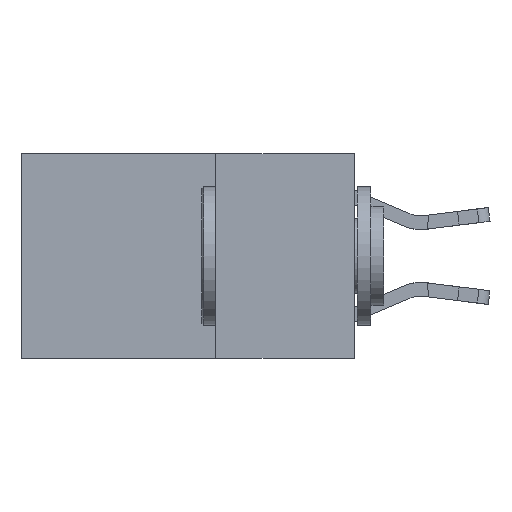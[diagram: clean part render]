
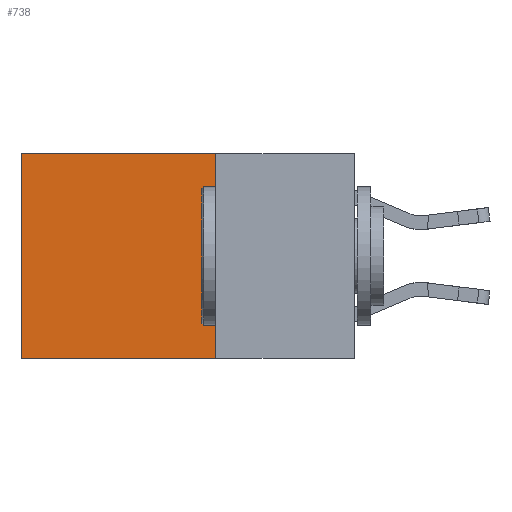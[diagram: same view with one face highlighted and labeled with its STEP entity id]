
A CAD part, left-side view. The second image highlights one B-rep face of the part: STEP entity #738.
In plain terms, the highlighted planar face has unit normal (-1, 0, 0).
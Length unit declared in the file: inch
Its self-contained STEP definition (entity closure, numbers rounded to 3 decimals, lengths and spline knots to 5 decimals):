
#284 = VERTEX_POINT ( 'NONE', #6397 ) ;
#473 = EDGE_LOOP ( 'NONE', ( #6124, #10874, #9040, #774 ) ) ;
#738 = ADVANCED_FACE ( 'NONE', ( #1685 ), #13209, .F. ) ;
#774 = ORIENTED_EDGE ( 'NONE', *, *, #2494, .T. ) ;
#1008 = CARTESIAN_POINT ( 'NONE',  ( 0.2625, 0.6, -0.37 ) ) ;
#1358 = DIRECTION ( 'NONE',  ( 0., 0., -1. ) ) ;
#1457 = CARTESIAN_POINT ( 'NONE',  ( 0.2625, 0.6, 0. ) ) ;
#1685 = FACE_OUTER_BOUND ( 'NONE', #473, .T. ) ;
#2107 = EDGE_CURVE ( 'NONE', #284, #2161, #4138, .T. ) ;
#2161 = VERTEX_POINT ( 'NONE', #1008 ) ;
#2494 = EDGE_CURVE ( 'NONE', #5343, #284, #11928, .T. ) ;
#2899 = CARTESIAN_POINT ( 'NONE',  ( 0.2625, 0.25, 0. ) ) ;
#4138 = LINE ( 'NONE', #1457, #10422 ) ;
#4591 = CARTESIAN_POINT ( 'NONE',  ( 0.2625, 0.25, 0. ) ) ;
#5050 = EDGE_CURVE ( 'NONE', #7968, #2161, #9154, .T. ) ;
#5136 = CARTESIAN_POINT ( 'NONE',  ( 0.2625, 0.25, -0.37 ) ) ;
#5343 = VERTEX_POINT ( 'NONE', #4591 ) ;
#5575 = EDGE_CURVE ( 'NONE', #5343, #7968, #6940, .T. ) ;
#5639 = VECTOR ( 'NONE', #6352, 39.37008 ) ;
#6124 = ORIENTED_EDGE ( 'NONE', *, *, #2107, .T. ) ;
#6188 = CARTESIAN_POINT ( 'NONE',  ( 0.2625, 0.25, 0. ) ) ;
#6352 = DIRECTION ( 'NONE',  ( 0., 1., 0. ) ) ;
#6397 = CARTESIAN_POINT ( 'NONE',  ( 0.2625, 0.6, 0. ) ) ;
#6940 = LINE ( 'NONE', #6188, #12576 ) ;
#7968 = VERTEX_POINT ( 'NONE', #11797 ) ;
#9040 = ORIENTED_EDGE ( 'NONE', *, *, #5575, .F. ) ;
#9154 = LINE ( 'NONE', #5136, #5639 ) ;
#9714 = DIRECTION ( 'NONE',  ( 0., 0., -1. ) ) ;
#10422 = VECTOR ( 'NONE', #1358, 39.37008 ) ;
#10874 = ORIENTED_EDGE ( 'NONE', *, *, #5050, .F. ) ;
#11164 = DIRECTION ( 'NONE',  ( 0., 1., 0. ) ) ;
#11797 = CARTESIAN_POINT ( 'NONE',  ( 0.2625, 0.25, -0.37 ) ) ;
#11847 = AXIS2_PLACEMENT_3D ( 'NONE', #13282, #13139, #13119 ) ;
#11928 = LINE ( 'NONE', #2899, #12263 ) ;
#12263 = VECTOR ( 'NONE', #11164, 39.37008 ) ;
#12576 = VECTOR ( 'NONE', #9714, 39.37008 ) ;
#13119 = DIRECTION ( 'NONE',  ( 0., 0., -1. ) ) ;
#13139 = DIRECTION ( 'NONE',  ( 1., 0., 0. ) ) ;
#13209 = PLANE ( 'NONE',  #11847 ) ;
#13282 = CARTESIAN_POINT ( 'NONE',  ( 0.2625, 0.25, 0. ) ) ;
